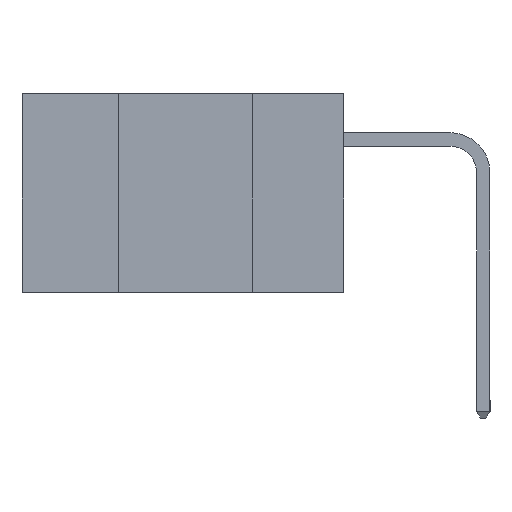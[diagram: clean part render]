
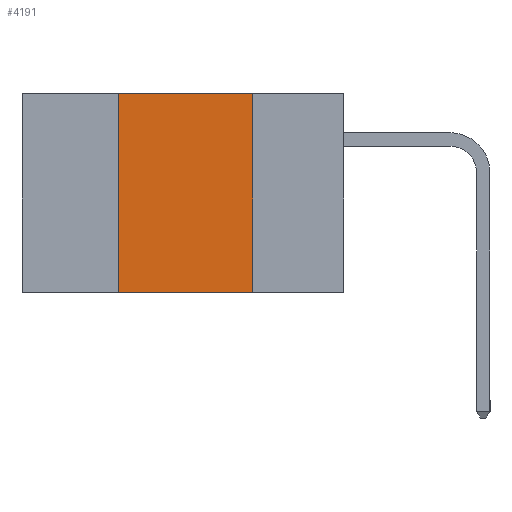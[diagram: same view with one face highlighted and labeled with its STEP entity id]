
A CAD part, left-side view. The second image highlights one B-rep face of the part: STEP entity #4191.
In plain terms, the highlighted planar face has unit normal (-1, 0, 0).
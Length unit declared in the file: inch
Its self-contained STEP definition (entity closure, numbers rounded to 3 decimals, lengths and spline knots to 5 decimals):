
#76 = LINE ( 'NONE', #2482, #2230 ) ;
#176 = LINE ( 'NONE', #5788, #8128 ) ;
#627 = EDGE_LOOP ( 'NONE', ( #6566, #10068, #4929, #12910 ) ) ;
#641 = EDGE_CURVE ( 'NONE', #9488, #9156, #5463, .T. ) ;
#1176 = VECTOR ( 'NONE', #3783, 39.37008 ) ;
#1355 = EDGE_CURVE ( 'NONE', #9156, #12226, #76, .T. ) ;
#1461 = DIRECTION ( 'NONE',  ( 0., 0., -1. ) ) ;
#1712 = VERTEX_POINT ( 'NONE', #2623 ) ;
#1723 = DIRECTION ( 'NONE',  ( 1., 0., 0. ) ) ;
#1733 = PLANE ( 'NONE',  #12667 ) ;
#2098 = CARTESIAN_POINT ( 'NONE',  ( 0., 0.6, 0. ) ) ;
#2230 = VECTOR ( 'NONE', #2390, 39.37008 ) ;
#2390 = DIRECTION ( 'NONE',  ( 0., -1., 0. ) ) ;
#2482 = CARTESIAN_POINT ( 'NONE',  ( 0., 0.6, 0. ) ) ;
#2623 = CARTESIAN_POINT ( 'NONE',  ( 0., 0.17, -0.37 ) ) ;
#3612 = CARTESIAN_POINT ( 'NONE',  ( 0., 0.17, -0.37 ) ) ;
#3707 = EDGE_CURVE ( 'NONE', #12226, #1712, #9399, .T. ) ;
#3783 = DIRECTION ( 'NONE',  ( 0., 0., -1. ) ) ;
#4191 = ADVANCED_FACE ( 'NONE', ( #8409 ), #1733, .F. ) ;
#4929 = ORIENTED_EDGE ( 'NONE', *, *, #641, .F. ) ;
#5463 = LINE ( 'NONE', #11040, #13087 ) ;
#5788 = CARTESIAN_POINT ( 'NONE',  ( 0., 0.6, -0.37 ) ) ;
#6566 = ORIENTED_EDGE ( 'NONE', *, *, #3707, .F. ) ;
#6857 = DIRECTION ( 'NONE',  ( 0., -1., 0. ) ) ;
#8128 = VECTOR ( 'NONE', #6857, 39.37008 ) ;
#8409 = FACE_OUTER_BOUND ( 'NONE', #627, .T. ) ;
#8868 = CARTESIAN_POINT ( 'NONE',  ( 0., 0.17, 0. ) ) ;
#9156 = VERTEX_POINT ( 'NONE', #10302 ) ;
#9399 = LINE ( 'NONE', #3612, #1176 ) ;
#9488 = VERTEX_POINT ( 'NONE', #11685 ) ;
#10068 = ORIENTED_EDGE ( 'NONE', *, *, #1355, .F. ) ;
#10302 = CARTESIAN_POINT ( 'NONE',  ( 0., 0.42, 0. ) ) ;
#11040 = CARTESIAN_POINT ( 'NONE',  ( 0., 0.42, -0.37 ) ) ;
#11132 = DIRECTION ( 'NONE',  ( 0., 0., 1. ) ) ;
#11685 = CARTESIAN_POINT ( 'NONE',  ( 0., 0.42, -0.37 ) ) ;
#12226 = VERTEX_POINT ( 'NONE', #8868 ) ;
#12667 = AXIS2_PLACEMENT_3D ( 'NONE', #2098, #1723, #1461 ) ;
#12910 = ORIENTED_EDGE ( 'NONE', *, *, #13088, .T. ) ;
#13087 = VECTOR ( 'NONE', #11132, 39.37008 ) ;
#13088 = EDGE_CURVE ( 'NONE', #9488, #1712, #176, .T. ) ;
